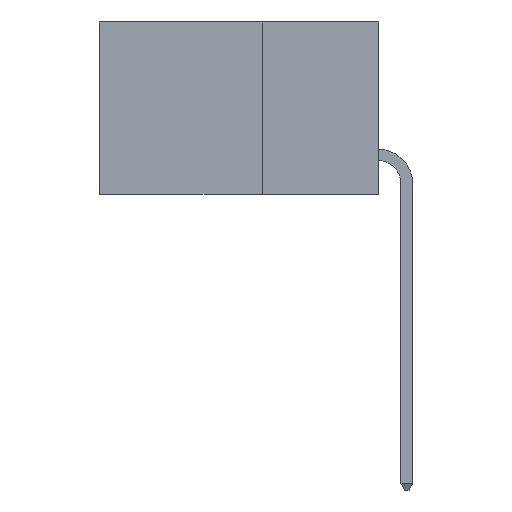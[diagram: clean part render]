
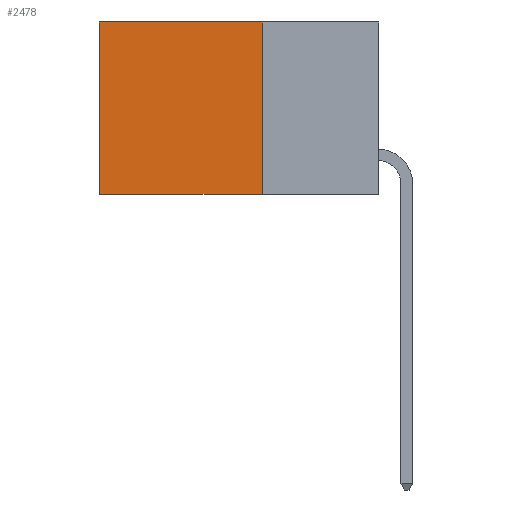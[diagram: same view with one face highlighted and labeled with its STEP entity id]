
A CAD part, left-side view. The second image highlights one B-rep face of the part: STEP entity #2478.
In plain terms, the highlighted planar face has unit normal (-1, 0, 0).
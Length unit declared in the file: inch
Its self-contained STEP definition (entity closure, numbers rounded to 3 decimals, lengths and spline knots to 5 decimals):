
#1067 = ORIENTED_EDGE ( 'NONE', *, *, #5757, .F. ) ;
#1150 = LINE ( 'NONE', #6045, #5747 ) ;
#1216 = CARTESIAN_POINT ( 'NONE',  ( 0.2615, 0.6, -0.37 ) ) ;
#1228 = VERTEX_POINT ( 'NONE', #7926 ) ;
#1358 = EDGE_CURVE ( 'NONE', #10912, #1894, #1150, .T. ) ;
#1894 = VERTEX_POINT ( 'NONE', #9887 ) ;
#1942 = DIRECTION ( 'NONE',  ( 0., 1., 0. ) ) ;
#2105 = DIRECTION ( 'NONE',  ( 0., 0., -1. ) ) ;
#2416 = DIRECTION ( 'NONE',  ( 0., 1., 0. ) ) ;
#2478 = ADVANCED_FACE ( 'NONE', ( #10542 ), #11145, .F. ) ;
#2732 = ORIENTED_EDGE ( 'NONE', *, *, #7321, .T. ) ;
#3027 = EDGE_LOOP ( 'NONE', ( #2732, #1067, #9727, #3725 ) ) ;
#3725 = ORIENTED_EDGE ( 'NONE', *, *, #4776, .T. ) ;
#4098 = VECTOR ( 'NONE', #2416, 39.37008 ) ;
#4776 = EDGE_CURVE ( 'NONE', #10912, #1228, #6581, .T. ) ;
#5747 = VECTOR ( 'NONE', #6021, 39.37008 ) ;
#5757 = EDGE_CURVE ( 'NONE', #1894, #5896, #10370, .T. ) ;
#5772 = CARTESIAN_POINT ( 'NONE',  ( 0.2615, 0.6, -0.37 ) ) ;
#5896 = VERTEX_POINT ( 'NONE', #5772 ) ;
#5949 = LINE ( 'NONE', #1216, #10353 ) ;
#5970 = VECTOR ( 'NONE', #1942, 39.37008 ) ;
#6021 = DIRECTION ( 'NONE',  ( 0., 0., -1. ) ) ;
#6045 = CARTESIAN_POINT ( 'NONE',  ( 0.2615, 0.25, -0.37 ) ) ;
#6561 = CARTESIAN_POINT ( 'NONE',  ( 0.2615, 0.25, -0.37 ) ) ;
#6581 = LINE ( 'NONE', #9655, #4098 ) ;
#7314 = CARTESIAN_POINT ( 'NONE',  ( 0.2615, 0.25, 0. ) ) ;
#7321 = EDGE_CURVE ( 'NONE', #1228, #5896, #5949, .T. ) ;
#7926 = CARTESIAN_POINT ( 'NONE',  ( 0.2615, 0.6, 0. ) ) ;
#9199 = AXIS2_PLACEMENT_3D ( 'NONE', #11113, #10886, #10874 ) ;
#9655 = CARTESIAN_POINT ( 'NONE',  ( 0.2615, 0.25, 0. ) ) ;
#9727 = ORIENTED_EDGE ( 'NONE', *, *, #1358, .F. ) ;
#9887 = CARTESIAN_POINT ( 'NONE',  ( 0.2615, 0.25, -0.37 ) ) ;
#10353 = VECTOR ( 'NONE', #2105, 39.37008 ) ;
#10370 = LINE ( 'NONE', #6561, #5970 ) ;
#10542 = FACE_OUTER_BOUND ( 'NONE', #3027, .T. ) ;
#10874 = DIRECTION ( 'NONE',  ( 0., 0., -1. ) ) ;
#10886 = DIRECTION ( 'NONE',  ( 1., 0., 0. ) ) ;
#10912 = VERTEX_POINT ( 'NONE', #7314 ) ;
#11113 = CARTESIAN_POINT ( 'NONE',  ( 0.2615, 0.25, -0.37 ) ) ;
#11145 = PLANE ( 'NONE',  #9199 ) ;
